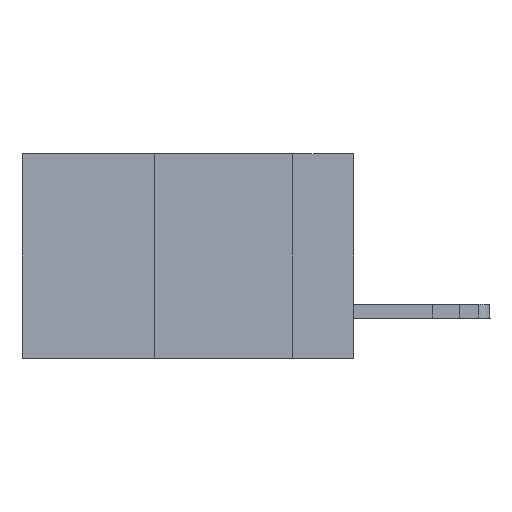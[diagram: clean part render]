
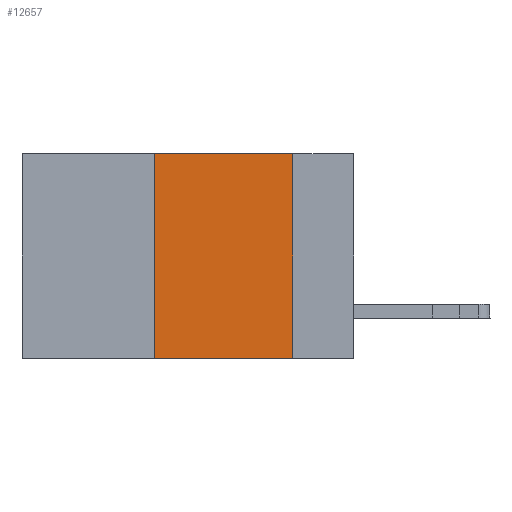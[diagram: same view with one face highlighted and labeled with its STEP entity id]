
A CAD part, left-side view. The second image highlights one B-rep face of the part: STEP entity #12657.
In plain terms, the highlighted planar face has unit normal (-1, 0, 0).
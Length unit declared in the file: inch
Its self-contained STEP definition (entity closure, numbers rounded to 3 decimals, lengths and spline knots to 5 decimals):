
#585 = CARTESIAN_POINT ( 'NONE',  ( 0., 0.36, 0. ) ) ;
#636 = VECTOR ( 'NONE', #12860, 39.37008 ) ;
#715 = AXIS2_PLACEMENT_3D ( 'NONE', #5617, #16256, #8400 ) ;
#1083 = CARTESIAN_POINT ( 'NONE',  ( 0., 0.11, 0. ) ) ;
#1107 = VECTOR ( 'NONE', #2134, 39.37008 ) ;
#1479 = PLANE ( 'NONE',  #715 ) ;
#2134 = DIRECTION ( 'NONE',  ( 0., -1., 0. ) ) ;
#2217 = VERTEX_POINT ( 'NONE', #11437 ) ;
#2831 = CARTESIAN_POINT ( 'NONE',  ( 0., 0.36, 0. ) ) ;
#2845 = ORIENTED_EDGE ( 'NONE', *, *, #10337, .F. ) ;
#3709 = ORIENTED_EDGE ( 'NONE', *, *, #14183, .T. ) ;
#4624 = EDGE_CURVE ( 'NONE', #15009, #7827, #7131, .T. ) ;
#4775 = VERTEX_POINT ( 'NONE', #14383 ) ;
#5617 = CARTESIAN_POINT ( 'NONE',  ( 0., 0.6, 0. ) ) ;
#5792 = EDGE_CURVE ( 'NONE', #4775, #15009, #7938, .T. ) ;
#7131 = LINE ( 'NONE', #11543, #636 ) ;
#7496 = VECTOR ( 'NONE', #15362, 39.37008 ) ;
#7827 = VERTEX_POINT ( 'NONE', #1083 ) ;
#7938 = LINE ( 'NONE', #585, #7496 ) ;
#8400 = DIRECTION ( 'NONE',  ( 0., 0., -1. ) ) ;
#8475 = CARTESIAN_POINT ( 'NONE',  ( 0., 0.11, 0. ) ) ;
#8967 = CARTESIAN_POINT ( 'NONE',  ( 0., 0.6, -0.37 ) ) ;
#10337 = EDGE_CURVE ( 'NONE', #7827, #2217, #12695, .T. ) ;
#11110 = EDGE_LOOP ( 'NONE', ( #2845, #13617, #17041, #3709 ) ) ;
#11138 = DIRECTION ( 'NONE',  ( 0., 0., -1. ) ) ;
#11437 = CARTESIAN_POINT ( 'NONE',  ( 0., 0.11, -0.37 ) ) ;
#11543 = CARTESIAN_POINT ( 'NONE',  ( 0., 0.6, 0. ) ) ;
#12657 = ADVANCED_FACE ( 'NONE', ( #13459 ), #1479, .F. ) ;
#12695 = LINE ( 'NONE', #8475, #15723 ) ;
#12860 = DIRECTION ( 'NONE',  ( 0., -1., 0. ) ) ;
#13459 = FACE_OUTER_BOUND ( 'NONE', #11110, .T. ) ;
#13617 = ORIENTED_EDGE ( 'NONE', *, *, #4624, .F. ) ;
#14183 = EDGE_CURVE ( 'NONE', #4775, #2217, #15402, .T. ) ;
#14383 = CARTESIAN_POINT ( 'NONE',  ( 0., 0.36, -0.37 ) ) ;
#15009 = VERTEX_POINT ( 'NONE', #2831 ) ;
#15362 = DIRECTION ( 'NONE',  ( 0., 0., 1. ) ) ;
#15402 = LINE ( 'NONE', #8967, #1107 ) ;
#15723 = VECTOR ( 'NONE', #11138, 39.37008 ) ;
#16256 = DIRECTION ( 'NONE',  ( 1., 0., 0. ) ) ;
#17041 = ORIENTED_EDGE ( 'NONE', *, *, #5792, .F. ) ;
